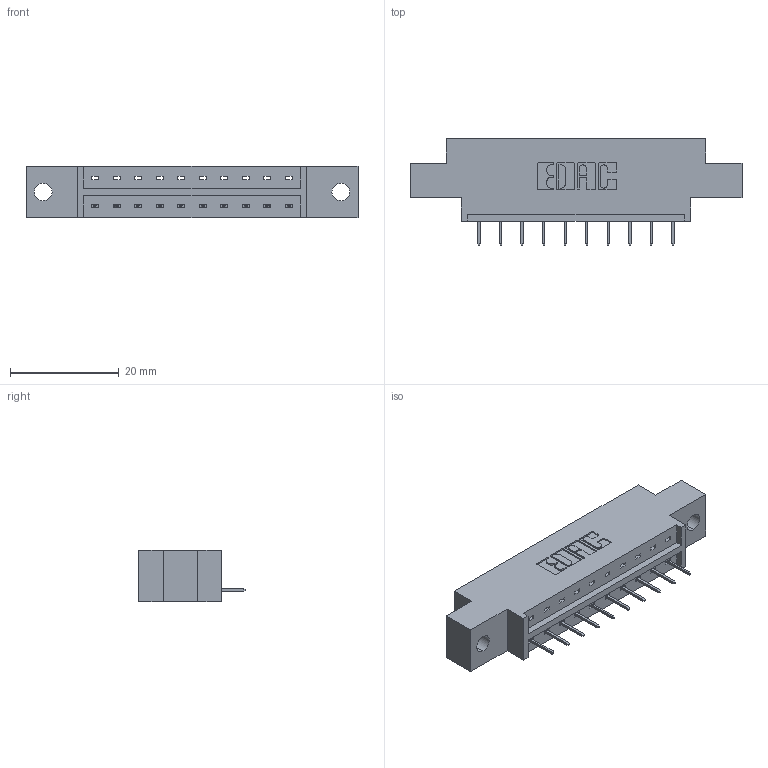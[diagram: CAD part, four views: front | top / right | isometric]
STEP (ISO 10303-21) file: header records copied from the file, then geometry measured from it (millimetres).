
FILE_DESCRIPTION (( 'STEP AP203' ), '1' );
FILE_NAME ('833-010-524-602.STEP', '2020-05-30T18:27:20', ( '' ), ( '' ), 'SwSTEP 2.0', 'SolidWorks 2020', '' );
FILE_SCHEMA (( 'CONFIG_CONTROL_DESIGN' ));
Length unit declared in the file: inch
Products named in the file (3): 833 Part_Offset - .128 Dia; 345-292-001_345-293-124; 833-010-524-602
Assembly tree (11 placements, depth 2):
  833-010-524-602
    833 Part_Offset - .128 Dia
    345-292-001_345-293-124  x10
Bounding box: 61.16 x 19.69 x 9.4 mm (x, y, z)
Volume: 5575.6 mm3; surface area: 5613.2 mm2
Topology: 11 solids, 11 shells, 738 faces, 2123 edges, 1374 vertices
Faces by surface type: plane 554, cylinder 184
Entity records: 10461 total; most frequent: CARTESIAN_POINT 1816, ORIENTED_EDGE 1762, DIRECTION 1597, EDGE_CURVE 881, VECTOR 757, LINE 757, VERTEX_POINT 582, AXIS2_PLACEMENT_3D 420
